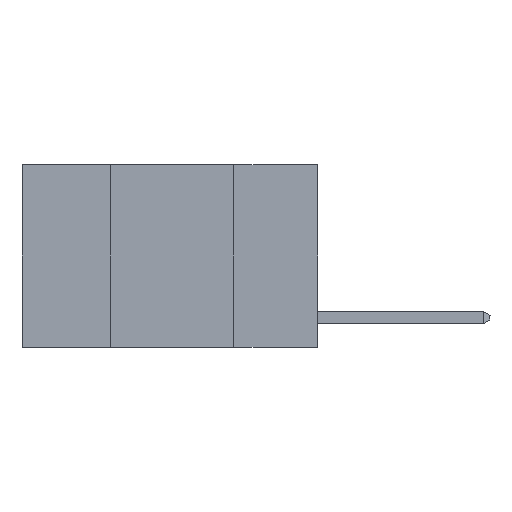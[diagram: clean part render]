
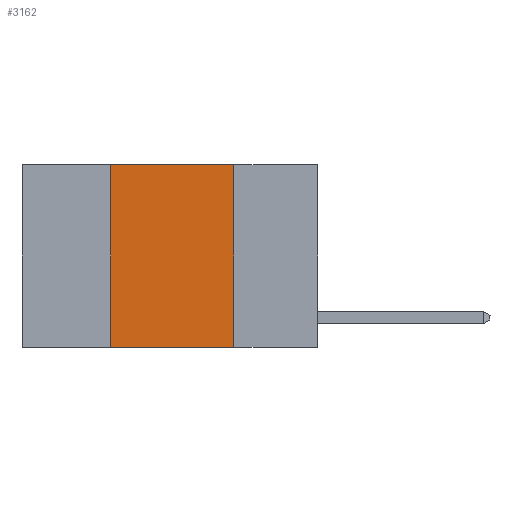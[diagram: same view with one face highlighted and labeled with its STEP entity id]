
A CAD part, left-side view. The second image highlights one B-rep face of the part: STEP entity #3162.
In plain terms, the highlighted planar face has unit normal (-1, 0, 0).
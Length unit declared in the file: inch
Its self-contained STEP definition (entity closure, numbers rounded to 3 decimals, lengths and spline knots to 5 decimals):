
#332 = CARTESIAN_POINT ( 'NONE',  ( 0., 0.6, 0. ) ) ;
#383 = DIRECTION ( 'NONE',  ( 0., -1., 0. ) ) ;
#730 = CARTESIAN_POINT ( 'NONE',  ( 0., 0.6, 0. ) ) ;
#940 = LINE ( 'NONE', #4282, #10816 ) ;
#1354 = LINE ( 'NONE', #8047, #4721 ) ;
#1697 = ORIENTED_EDGE ( 'NONE', *, *, #11924, .F. ) ;
#1754 = CARTESIAN_POINT ( 'NONE',  ( 0., 0.42, 0. ) ) ;
#1821 = DIRECTION ( 'NONE',  ( 0., 0., -1. ) ) ;
#2458 = LINE ( 'NONE', #9244, #10946 ) ;
#2501 = DIRECTION ( 'NONE',  ( 0., -1., 0. ) ) ;
#2560 = EDGE_LOOP ( 'NONE', ( #1697, #8045, #13332, #3443 ) ) ;
#2637 = CARTESIAN_POINT ( 'NONE',  ( 0., 0.42, -0.37 ) ) ;
#2669 = EDGE_CURVE ( 'NONE', #10257, #8112, #1354, .T. ) ;
#2753 = LINE ( 'NONE', #332, #8460 ) ;
#3162 = ADVANCED_FACE ( 'NONE', ( #9765 ), #7199, .F. ) ;
#3443 = ORIENTED_EDGE ( 'NONE', *, *, #2669, .T. ) ;
#4011 = EDGE_CURVE ( 'NONE', #9264, #8120, #2753, .T. ) ;
#4282 = CARTESIAN_POINT ( 'NONE',  ( 0., 0.42, 0. ) ) ;
#4721 = VECTOR ( 'NONE', #383, 39.37008 ) ;
#5135 = DIRECTION ( 'NONE',  ( 0., 0., 1. ) ) ;
#7105 = DIRECTION ( 'NONE',  ( 1., 0., 0. ) ) ;
#7199 = PLANE ( 'NONE',  #11101 ) ;
#8045 = ORIENTED_EDGE ( 'NONE', *, *, #4011, .F. ) ;
#8047 = CARTESIAN_POINT ( 'NONE',  ( 0., 0.6, -0.37 ) ) ;
#8112 = VERTEX_POINT ( 'NONE', #12005 ) ;
#8120 = VERTEX_POINT ( 'NONE', #13074 ) ;
#8460 = VECTOR ( 'NONE', #2501, 39.37008 ) ;
#9244 = CARTESIAN_POINT ( 'NONE',  ( 0., 0.17, 0. ) ) ;
#9264 = VERTEX_POINT ( 'NONE', #1754 ) ;
#9765 = FACE_OUTER_BOUND ( 'NONE', #2560, .T. ) ;
#10257 = VERTEX_POINT ( 'NONE', #2637 ) ;
#10816 = VECTOR ( 'NONE', #5135, 39.37008 ) ;
#10946 = VECTOR ( 'NONE', #11324, 39.37008 ) ;
#11078 = EDGE_CURVE ( 'NONE', #10257, #9264, #940, .T. ) ;
#11101 = AXIS2_PLACEMENT_3D ( 'NONE', #730, #7105, #1821 ) ;
#11324 = DIRECTION ( 'NONE',  ( 0., 0., -1. ) ) ;
#11924 = EDGE_CURVE ( 'NONE', #8120, #8112, #2458, .T. ) ;
#12005 = CARTESIAN_POINT ( 'NONE',  ( 0., 0.17, -0.37 ) ) ;
#13074 = CARTESIAN_POINT ( 'NONE',  ( 0., 0.17, 0. ) ) ;
#13332 = ORIENTED_EDGE ( 'NONE', *, *, #11078, .F. ) ;
